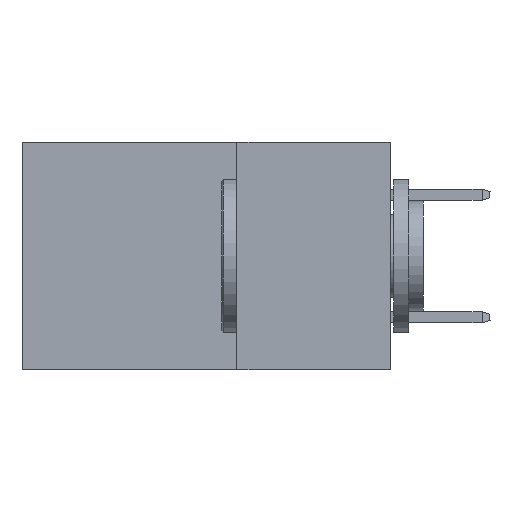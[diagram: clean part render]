
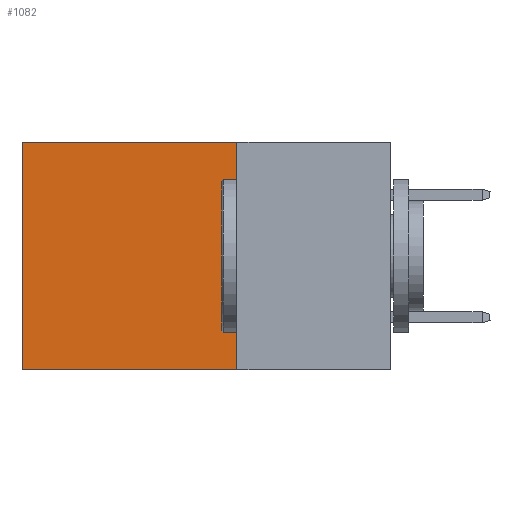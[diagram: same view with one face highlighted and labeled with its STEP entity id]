
A CAD part, left-side view. The second image highlights one B-rep face of the part: STEP entity #1082.
In plain terms, the highlighted planar face has unit normal (-1, 0, 0).
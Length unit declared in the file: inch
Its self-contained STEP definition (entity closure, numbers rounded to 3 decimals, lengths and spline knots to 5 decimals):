
#169 = DIRECTION ( 'NONE',  ( 1., 0., 0. ) ) ;
#1082 = ADVANCED_FACE ( 'NONE', ( #17787 ), #12971, .F. ) ;
#1108 = CARTESIAN_POINT ( 'NONE',  ( 0.2875, 0.25, 0. ) ) ;
#1190 = ORIENTED_EDGE ( 'NONE', *, *, #7993, .T. ) ;
#2320 = CARTESIAN_POINT ( 'NONE',  ( 0.2875, 0.6, 0. ) ) ;
#2462 = VECTOR ( 'NONE', #7259, 39.37008 ) ;
#2472 = CARTESIAN_POINT ( 'NONE',  ( 0.2875, 0.25, 0. ) ) ;
#2642 = VERTEX_POINT ( 'NONE', #7687 ) ;
#3006 = DIRECTION ( 'NONE',  ( 0., 0., -1. ) ) ;
#3386 = VERTEX_POINT ( 'NONE', #13811 ) ;
#3853 = EDGE_CURVE ( 'NONE', #16565, #3386, #17335, .T. ) ;
#3895 = EDGE_CURVE ( 'NONE', #2642, #3386, #16462, .T. ) ;
#4085 = VECTOR ( 'NONE', #5551, 39.37008 ) ;
#5444 = AXIS2_PLACEMENT_3D ( 'NONE', #9896, #169, #14373 ) ;
#5527 = ORIENTED_EDGE ( 'NONE', *, *, #3895, .F. ) ;
#5551 = DIRECTION ( 'NONE',  ( 0., 1., 0. ) ) ;
#5679 = CARTESIAN_POINT ( 'NONE',  ( 0.2875, 0.25, -0.37 ) ) ;
#6893 = CARTESIAN_POINT ( 'NONE',  ( 0.2875, 0.25, 0. ) ) ;
#7259 = DIRECTION ( 'NONE',  ( 0., 1., 0. ) ) ;
#7458 = ORIENTED_EDGE ( 'NONE', *, *, #3853, .T. ) ;
#7687 = CARTESIAN_POINT ( 'NONE',  ( 0.2875, 0.25, -0.37 ) ) ;
#7975 = CARTESIAN_POINT ( 'NONE',  ( 0.2875, 0.6, 0. ) ) ;
#7993 = EDGE_CURVE ( 'NONE', #8104, #16565, #11558, .T. ) ;
#8104 = VERTEX_POINT ( 'NONE', #1108 ) ;
#9273 = LINE ( 'NONE', #2472, #10129 ) ;
#9350 = EDGE_LOOP ( 'NONE', ( #7458, #5527, #13131, #1190 ) ) ;
#9488 = VECTOR ( 'NONE', #12158, 39.37008 ) ;
#9896 = CARTESIAN_POINT ( 'NONE',  ( 0.2875, 0.25, 0. ) ) ;
#10129 = VECTOR ( 'NONE', #3006, 39.37008 ) ;
#10976 = EDGE_CURVE ( 'NONE', #8104, #2642, #9273, .T. ) ;
#11558 = LINE ( 'NONE', #6893, #4085 ) ;
#12158 = DIRECTION ( 'NONE',  ( 0., 0., -1. ) ) ;
#12971 = PLANE ( 'NONE',  #5444 ) ;
#13131 = ORIENTED_EDGE ( 'NONE', *, *, #10976, .F. ) ;
#13811 = CARTESIAN_POINT ( 'NONE',  ( 0.2875, 0.6, -0.37 ) ) ;
#14373 = DIRECTION ( 'NONE',  ( 0., 0., -1. ) ) ;
#16462 = LINE ( 'NONE', #5679, #2462 ) ;
#16565 = VERTEX_POINT ( 'NONE', #2320 ) ;
#17335 = LINE ( 'NONE', #7975, #9488 ) ;
#17787 = FACE_OUTER_BOUND ( 'NONE', #9350, .T. ) ;
